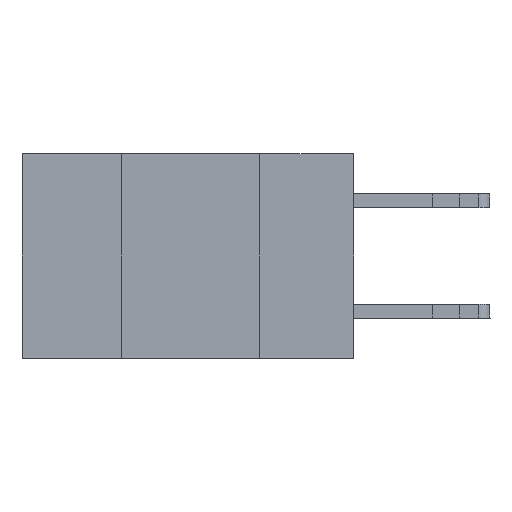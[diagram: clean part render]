
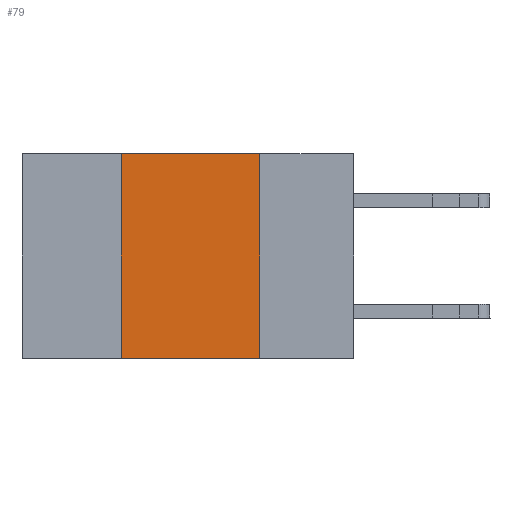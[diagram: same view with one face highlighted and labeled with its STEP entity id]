
A CAD part, left-side view. The second image highlights one B-rep face of the part: STEP entity #79.
In plain terms, the highlighted planar face has unit normal (-1, 0, 0).
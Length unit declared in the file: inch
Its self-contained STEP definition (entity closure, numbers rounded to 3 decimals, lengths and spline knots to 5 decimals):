
#79 = ADVANCED_FACE ( 'NONE', ( #1576 ), #15292, .F. ) ;
#338 = DIRECTION ( 'NONE',  ( 0., -1., 0. ) ) ;
#492 = LINE ( 'NONE', #20562, #21854 ) ;
#1029 = VERTEX_POINT ( 'NONE', #9805 ) ;
#1576 = FACE_OUTER_BOUND ( 'NONE', #11155, .T. ) ;
#2704 = VECTOR ( 'NONE', #19007, 39.37008 ) ;
#2743 = VERTEX_POINT ( 'NONE', #9717 ) ;
#3225 = ORIENTED_EDGE ( 'NONE', *, *, #21111, .F. ) ;
#3991 = VERTEX_POINT ( 'NONE', #20796 ) ;
#4265 = ORIENTED_EDGE ( 'NONE', *, *, #8302, .T. ) ;
#4842 = AXIS2_PLACEMENT_3D ( 'NONE', #14268, #18879, #21175 ) ;
#4942 = EDGE_CURVE ( 'NONE', #11020, #2743, #12584, .T. ) ;
#6004 = LINE ( 'NONE', #6827, #14990 ) ;
#6657 = ORIENTED_EDGE ( 'NONE', *, *, #4942, .F. ) ;
#6827 = CARTESIAN_POINT ( 'NONE',  ( 0., 0.17, 0. ) ) ;
#7195 = LINE ( 'NONE', #13975, #2704 ) ;
#8172 = VECTOR ( 'NONE', #10815, 39.37008 ) ;
#8302 = EDGE_CURVE ( 'NONE', #11020, #1029, #7195, .T. ) ;
#9717 = CARTESIAN_POINT ( 'NONE',  ( 0., 0.42, 0. ) ) ;
#9805 = CARTESIAN_POINT ( 'NONE',  ( 0., 0.17, -0.37 ) ) ;
#10815 = DIRECTION ( 'NONE',  ( 0., 0., 1. ) ) ;
#11020 = VERTEX_POINT ( 'NONE', #17645 ) ;
#11155 = EDGE_LOOP ( 'NONE', ( #3225, #19518, #6657, #4265 ) ) ;
#11259 = CARTESIAN_POINT ( 'NONE',  ( 0., 0.42, 0. ) ) ;
#12584 = LINE ( 'NONE', #11259, #8172 ) ;
#13471 = EDGE_CURVE ( 'NONE', #2743, #3991, #492, .T. ) ;
#13975 = CARTESIAN_POINT ( 'NONE',  ( 0., 0.6, -0.37 ) ) ;
#14268 = CARTESIAN_POINT ( 'NONE',  ( 0., 0.6, 0. ) ) ;
#14990 = VECTOR ( 'NONE', #15304, 39.37008 ) ;
#15292 = PLANE ( 'NONE',  #4842 ) ;
#15304 = DIRECTION ( 'NONE',  ( 0., 0., -1. ) ) ;
#17645 = CARTESIAN_POINT ( 'NONE',  ( 0., 0.42, -0.37 ) ) ;
#18879 = DIRECTION ( 'NONE',  ( 1., 0., 0. ) ) ;
#19007 = DIRECTION ( 'NONE',  ( 0., -1., 0. ) ) ;
#19518 = ORIENTED_EDGE ( 'NONE', *, *, #13471, .F. ) ;
#20562 = CARTESIAN_POINT ( 'NONE',  ( 0., 0.6, 0. ) ) ;
#20796 = CARTESIAN_POINT ( 'NONE',  ( 0., 0.17, 0. ) ) ;
#21111 = EDGE_CURVE ( 'NONE', #3991, #1029, #6004, .T. ) ;
#21175 = DIRECTION ( 'NONE',  ( 0., 0., -1. ) ) ;
#21854 = VECTOR ( 'NONE', #338, 39.37008 ) ;
